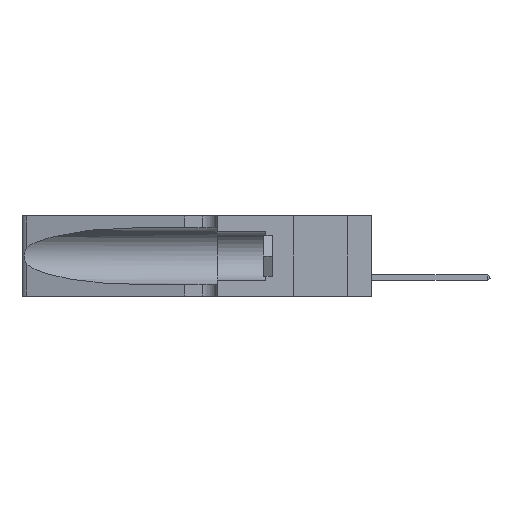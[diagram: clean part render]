
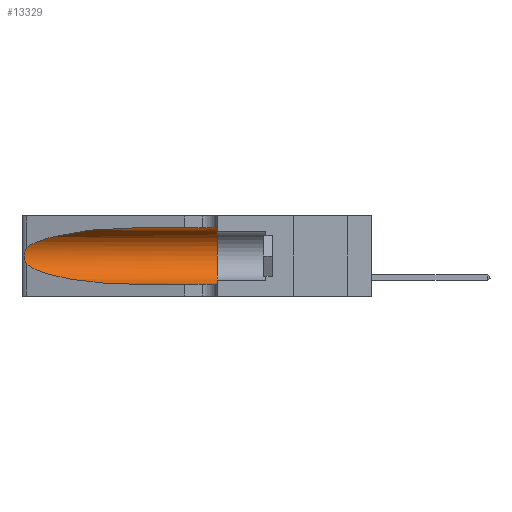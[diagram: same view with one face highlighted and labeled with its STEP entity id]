
A CAD part, left-side view. The second image highlights one B-rep face of the part: STEP entity #13329.
In plain terms, the highlighted cylindrical face has radius 3.308 mm (diameter 6.617 mm), a partial arc.
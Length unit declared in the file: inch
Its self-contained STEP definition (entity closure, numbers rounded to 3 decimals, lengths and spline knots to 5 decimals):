
#434 = CARTESIAN_POINT ( 'NONE',  ( 0.25854, 1.2359, 0.20912 ) ) ;
#708 = CARTESIAN_POINT ( 'NONE',  ( 0.2373, 1.15595, 0.08982 ) ) ;
#1247 = CARTESIAN_POINT ( 'NONE',  ( 0.26075, 1.23896, 0.178 ) ) ;
#2450 = EDGE_CURVE ( 'NONE', #32681, #3443, #29690, .T. ) ;
#3443 = VERTEX_POINT ( 'NONE', #12352 ) ;
#3668 = ORIENTED_EDGE ( 'NONE', *, *, #28443, .F. ) ;
#4195 = CARTESIAN_POINT ( 'NONE',  ( 0.25487, 1.22718, 0.14631 ) ) ;
#5276 = ORIENTED_EDGE ( 'NONE', *, *, #28582, .T. ) ;
#5393 = CARTESIAN_POINT ( 'NONE',  ( 0.2373, 1.15595, 0.28018 ) ) ;
#5435 = CARTESIAN_POINT ( 'NONE',  ( 0.25487, 1.22718, 0.14631 ) ) ;
#6420 = CARTESIAN_POINT ( 'NONE',  ( 0.1305, 0.35, 0.185 ) ) ;
#6799 = CARTESIAN_POINT ( 'NONE',  ( 0.1305, 0.72297, 0.31525 ) ) ;
#7166 = VERTEX_POINT ( 'NONE', #6799 ) ;
#7286 = CARTESIAN_POINT ( 'NONE',  ( 0.25555, 1.22994, 0.2215 ) ) ;
#7891 = CYLINDRICAL_SURFACE ( 'NONE', #24118, 0.13025 ) ;
#9146 = CARTESIAN_POINT ( 'NONE',  ( 0.25555, 1.22993, 0.14849 ) ) ;
#11232 = CARTESIAN_POINT ( 'NONE',  ( 0.26075, 1.23896, 0.19203 ) ) ;
#11410 = CARTESIAN_POINT ( 'NONE',  ( 0.1305, 1.61858, 0.185 ) ) ;
#11726 = DIRECTION ( 'NONE',  ( 0., -1., 0. ) ) ;
#11765 = VERTEX_POINT ( 'NONE', #20248 ) ;
#12352 = CARTESIAN_POINT ( 'NONE',  ( 0.1305, 0.35, 0.05475 ) ) ;
#12480 = EDGE_LOOP ( 'NONE', ( #31113, #5276, #24131, #20458, #3668, #16126 ) ) ;
#13329 = ADVANCED_FACE ( 'NONE', ( #18618 ), #7891, .F. ) ;
#15427 = CARTESIAN_POINT ( 'NONE',  ( 0.25487, 1.22718, 0.22369 ) ) ;
#16126 = ORIENTED_EDGE ( 'NONE', *, *, #20312, .F. ) ;
#16728 = DIRECTION ( 'NONE',  ( 0., 0., 1. ) ) ;
#17202 = DIRECTION ( 'NONE',  ( 0., 1., 0. ) ) ;
#17285 = DIRECTION ( 'NONE',  ( 0., -1., 0. ) ) ;
#18079 = CARTESIAN_POINT ( 'NONE',  ( 0.26018, 1.23835, 0.19895 ) ) ;
#18340 = CARTESIAN_POINT ( 'NONE',  ( 0.1305, 0.72297, 0.05475 ) ) ;
#18618 = FACE_OUTER_BOUND ( 'NONE', #12480, .T. ) ;
#19308 = CARTESIAN_POINT ( 'NONE',  ( 0.25639, 1.23186, 0.15144 ) ) ;
#19530 =( BOUNDED_CURVE ( )  B_SPLINE_CURVE ( 3, ( #30541, #20479, #5393, #28086 ),
 .UNSPECIFIED., .F., .F. ) 
 B_SPLINE_CURVE_WITH_KNOTS ( ( 4, 4 ),
 ( 1.5708, 2.84003 ),
 .UNSPECIFIED. ) 
 CURVE ( )  GEOMETRIC_REPRESENTATION_ITEM ( )  RATIONAL_B_SPLINE_CURVE ( ( 1., 0.87, 0.87, 1. ) ) 
 REPRESENTATION_ITEM ( '' )  );
#19612 = CARTESIAN_POINT ( 'NONE',  ( 0.26017, 1.23833, 0.17102 ) ) ;
#19925 = CARTESIAN_POINT ( 'NONE',  ( 0.1305, 1.61858, 0.31525 ) ) ;
#20143 = CIRCLE ( 'NONE', #21650, 0.13025 ) ;
#20248 = CARTESIAN_POINT ( 'NONE',  ( 0.1305, 0.35, 0.31525 ) ) ;
#20312 = EDGE_CURVE ( 'NONE', #7166, #11765, #27126, .T. ) ;
#20458 = ORIENTED_EDGE ( 'NONE', *, *, #2450, .T. ) ;
#20479 = CARTESIAN_POINT ( 'NONE',  ( 0.18966, 0.96281, 0.31525 ) ) ;
#21650 = AXIS2_PLACEMENT_3D ( 'NONE', #6420, #17202, #16728 ) ;
#21724 = CARTESIAN_POINT ( 'NONE',  ( 0.25789, 1.23486, 0.15765 ) ) ;
#22711 = VERTEX_POINT ( 'NONE', #22960 ) ;
#22874 = CARTESIAN_POINT ( 'NONE',  ( 0.1305, 1.61858, 0.05475 ) ) ;
#22960 = CARTESIAN_POINT ( 'NONE',  ( 0.25487, 1.22718, 0.14631 ) ) ;
#23566 = VERTEX_POINT ( 'NONE', #15427 ) ;
#23594 = CARTESIAN_POINT ( 'NONE',  ( 0.25787, 1.23484, 0.2124 ) ) ;
#23598 = VECTOR ( 'NONE', #17285, 39.37008 ) ;
#24118 = AXIS2_PLACEMENT_3D ( 'NONE', #11410, #11726, #25922 ) ;
#24131 = ORIENTED_EDGE ( 'NONE', *, *, #25200, .T. ) ;
#24889 = DIRECTION ( 'NONE',  ( 0., -1., 0. ) ) ;
#25200 = EDGE_CURVE ( 'NONE', #22711, #32681, #25971, .T. ) ;
#25897 = CARTESIAN_POINT ( 'NONE',  ( 0.25639, 1.23184, 0.21858 ) ) ;
#25922 = DIRECTION ( 'NONE',  ( 0., 0., -1. ) ) ;
#25971 =( BOUNDED_CURVE ( )  B_SPLINE_CURVE ( 3, ( #5435, #708, #28471, #18340 ),
 .UNSPECIFIED., .F., .F. ) 
 B_SPLINE_CURVE_WITH_KNOTS ( ( 4, 4 ),
 ( 3.44316, 4.71239 ),
 .UNSPECIFIED. ) 
 CURVE ( )  GEOMETRIC_REPRESENTATION_ITEM ( )  RATIONAL_B_SPLINE_CURVE ( ( 1., 0.87, 0.87, 1. ) ) 
 REPRESENTATION_ITEM ( '' )  );
#26526 = VECTOR ( 'NONE', #24889, 39.37008 ) ;
#27126 = LINE ( 'NONE', #19925, #23598 ) ;
#28086 = CARTESIAN_POINT ( 'NONE',  ( 0.25487, 1.22718, 0.22369 ) ) ;
#28443 = EDGE_CURVE ( 'NONE', #11765, #3443, #20143, .T. ) ;
#28471 = CARTESIAN_POINT ( 'NONE',  ( 0.18966, 0.96281, 0.05475 ) ) ;
#28582 = EDGE_CURVE ( 'NONE', #23566, #22711, #32272, .T. ) ;
#28831 = CARTESIAN_POINT ( 'NONE',  ( 0.1305, 0.72297, 0.05475 ) ) ;
#29690 = LINE ( 'NONE', #22874, #26526 ) ;
#30541 = CARTESIAN_POINT ( 'NONE',  ( 0.1305, 0.72297, 0.31525 ) ) ;
#30685 = EDGE_CURVE ( 'NONE', #7166, #23566, #19530, .T. ) ;
#31113 = ORIENTED_EDGE ( 'NONE', *, *, #30685, .T. ) ;
#32077 = CARTESIAN_POINT ( 'NONE',  ( 0.25856, 1.23593, 0.16098 ) ) ;
#32272 = B_SPLINE_CURVE_WITH_KNOTS ( 'NONE', 3,
 ( #32438, #7286, #25897, #23594, #434, #18079, #11232, #1247, #19612, #32077, #21724, #19308, #9146, #4195 ),
 .UNSPECIFIED., .F., .F.,
 ( 4, 2, 2, 2, 2, 2, 4 ),
 ( 0., 0.00027, 0.00053, 0.00107, 0.0016, 0.00187, 0.00214 ),
 .UNSPECIFIED. ) ;
#32438 = CARTESIAN_POINT ( 'NONE',  ( 0.25487, 1.22718, 0.22369 ) ) ;
#32681 = VERTEX_POINT ( 'NONE', #28831 ) ;
